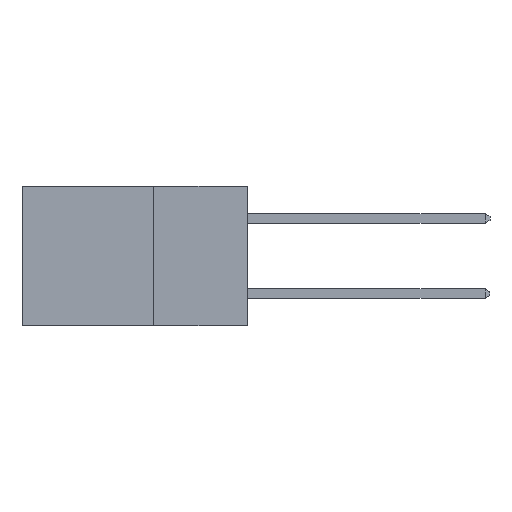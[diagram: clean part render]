
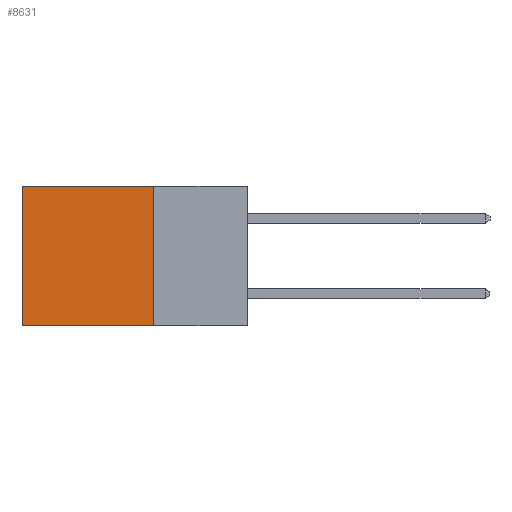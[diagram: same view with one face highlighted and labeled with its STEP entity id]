
A CAD part, left-side view. The second image highlights one B-rep face of the part: STEP entity #8631.
In plain terms, the highlighted planar face has unit normal (-1, 0, 0).
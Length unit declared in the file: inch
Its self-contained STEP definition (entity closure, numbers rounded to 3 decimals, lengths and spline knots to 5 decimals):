
#1536 = ORIENTED_EDGE ( 'NONE', *, *, #6447, .T. ) ;
#1854 = EDGE_LOOP ( 'NONE', ( #1536, #10181, #9676, #5952 ) ) ;
#2819 = DIRECTION ( 'NONE',  ( 0., 0., -1. ) ) ;
#2907 = EDGE_CURVE ( 'NONE', #16897, #26394, #22833, .T. ) ;
#2954 = DIRECTION ( 'NONE',  ( 0., 1., 0. ) ) ;
#3107 = DIRECTION ( 'NONE',  ( 1., 0., 0. ) ) ;
#3772 = CARTESIAN_POINT ( 'NONE',  ( 0.298, 0.6, 0. ) ) ;
#3938 = CARTESIAN_POINT ( 'NONE',  ( 0.298, 0.25, -0.37 ) ) ;
#5836 = VERTEX_POINT ( 'NONE', #3938 ) ;
#5952 = ORIENTED_EDGE ( 'NONE', *, *, #2907, .T. ) ;
#6210 = VECTOR ( 'NONE', #12392, 39.37008 ) ;
#6338 = VECTOR ( 'NONE', #2954, 39.37008 ) ;
#6447 = EDGE_CURVE ( 'NONE', #26394, #20357, #19152, .T. ) ;
#6805 = CARTESIAN_POINT ( 'NONE',  ( 0.298, 0.6, 0. ) ) ;
#8565 = EDGE_CURVE ( 'NONE', #16897, #5836, #21546, .T. ) ;
#8601 = AXIS2_PLACEMENT_3D ( 'NONE', #15616, #3107, #17655 ) ;
#8631 = ADVANCED_FACE ( 'NONE', ( #19642 ), #11449, .F. ) ;
#9676 = ORIENTED_EDGE ( 'NONE', *, *, #8565, .F. ) ;
#10181 = ORIENTED_EDGE ( 'NONE', *, *, #15542, .F. ) ;
#11449 = PLANE ( 'NONE',  #8601 ) ;
#12391 = VECTOR ( 'NONE', #2819, 39.37008 ) ;
#12392 = DIRECTION ( 'NONE',  ( 0., 1., 0. ) ) ;
#12475 = LINE ( 'NONE', #22587, #6210 ) ;
#15542 = EDGE_CURVE ( 'NONE', #5836, #20357, #12475, .T. ) ;
#15616 = CARTESIAN_POINT ( 'NONE',  ( 0.298, 0.25, 0. ) ) ;
#16897 = VERTEX_POINT ( 'NONE', #21137 ) ;
#17655 = DIRECTION ( 'NONE',  ( 0., 0., -1. ) ) ;
#19152 = LINE ( 'NONE', #6805, #12391 ) ;
#19559 = DIRECTION ( 'NONE',  ( 0., 0., -1. ) ) ;
#19642 = FACE_OUTER_BOUND ( 'NONE', #1854, .T. ) ;
#20357 = VERTEX_POINT ( 'NONE', #21436 ) ;
#20917 = VECTOR ( 'NONE', #19559, 39.37008 ) ;
#21137 = CARTESIAN_POINT ( 'NONE',  ( 0.298, 0.25, 0. ) ) ;
#21436 = CARTESIAN_POINT ( 'NONE',  ( 0.298, 0.6, -0.37 ) ) ;
#21546 = LINE ( 'NONE', #25580, #20917 ) ;
#22587 = CARTESIAN_POINT ( 'NONE',  ( 0.298, 0.25, -0.37 ) ) ;
#22833 = LINE ( 'NONE', #26011, #6338 ) ;
#25580 = CARTESIAN_POINT ( 'NONE',  ( 0.298, 0.25, 0. ) ) ;
#26011 = CARTESIAN_POINT ( 'NONE',  ( 0.298, 0.25, 0. ) ) ;
#26394 = VERTEX_POINT ( 'NONE', #3772 ) ;
